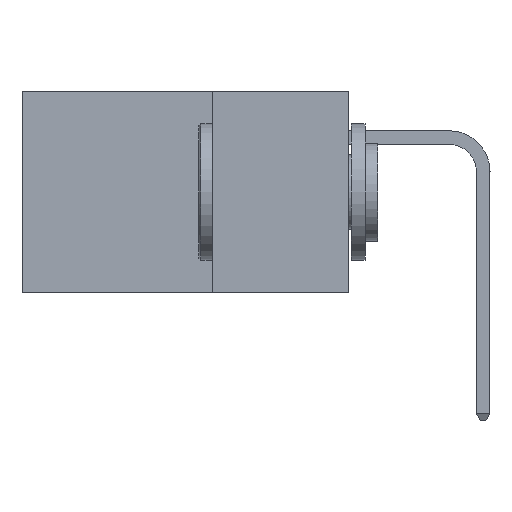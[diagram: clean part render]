
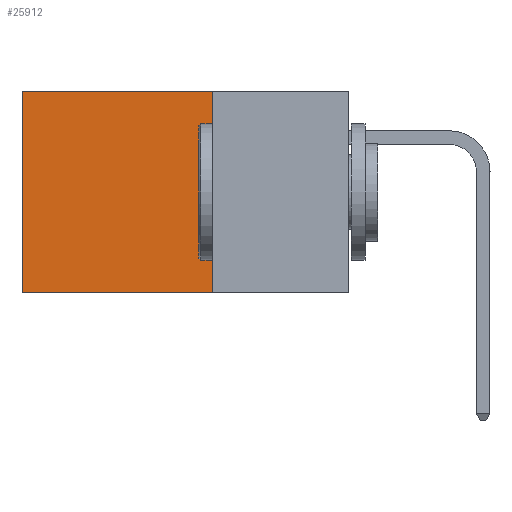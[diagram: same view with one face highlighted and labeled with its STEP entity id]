
A CAD part, left-side view. The second image highlights one B-rep face of the part: STEP entity #25912.
In plain terms, the highlighted planar face has unit normal (-1, 0, 0).
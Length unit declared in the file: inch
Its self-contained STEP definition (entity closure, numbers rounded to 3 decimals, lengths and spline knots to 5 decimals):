
#40 = FACE_OUTER_BOUND ( 'NONE', #26652, .T. ) ;
#1575 = CARTESIAN_POINT ( 'NONE',  ( 0.2875, 0.25, -0.37 ) ) ;
#2164 = VECTOR ( 'NONE', #14780, 39.37008 ) ;
#4225 = CARTESIAN_POINT ( 'NONE',  ( 0.2875, 0.6, 0. ) ) ;
#4243 = DIRECTION ( 'NONE',  ( 1., 0., 0. ) ) ;
#5872 = VERTEX_POINT ( 'NONE', #36141 ) ;
#5880 = VERTEX_POINT ( 'NONE', #33417 ) ;
#5999 = LINE ( 'NONE', #28860, #35302 ) ;
#6138 = VERTEX_POINT ( 'NONE', #14940 ) ;
#9954 = DIRECTION ( 'NONE',  ( 0., 0., -1. ) ) ;
#11559 = VECTOR ( 'NONE', #9954, 39.37008 ) ;
#11646 = ORIENTED_EDGE ( 'NONE', *, *, #27836, .F. ) ;
#11903 = CARTESIAN_POINT ( 'NONE',  ( 0.2875, 0.25, 0. ) ) ;
#14102 = LINE ( 'NONE', #1575, #28128 ) ;
#14710 = AXIS2_PLACEMENT_3D ( 'NONE', #21534, #4243, #24327 ) ;
#14780 = DIRECTION ( 'NONE',  ( 0., 0., -1. ) ) ;
#14940 = CARTESIAN_POINT ( 'NONE',  ( 0.2875, 0.25, 0. ) ) ;
#15315 = ORIENTED_EDGE ( 'NONE', *, *, #17483, .T. ) ;
#17483 = EDGE_CURVE ( 'NONE', #5872, #29052, #26513, .T. ) ;
#17976 = ORIENTED_EDGE ( 'NONE', *, *, #34341, .F. ) ;
#21534 = CARTESIAN_POINT ( 'NONE',  ( 0.2875, 0.25, 0. ) ) ;
#24327 = DIRECTION ( 'NONE',  ( 0., 0., -1. ) ) ;
#24574 = DIRECTION ( 'NONE',  ( 0., 1., 0. ) ) ;
#25063 = LINE ( 'NONE', #11903, #2164 ) ;
#25912 = ADVANCED_FACE ( 'NONE', ( #40 ), #29843, .F. ) ;
#26513 = LINE ( 'NONE', #4225, #11559 ) ;
#26652 = EDGE_LOOP ( 'NONE', ( #15315, #11646, #17976, #30438 ) ) ;
#27836 = EDGE_CURVE ( 'NONE', #5880, #29052, #14102, .T. ) ;
#28128 = VECTOR ( 'NONE', #24574, 39.37008 ) ;
#28860 = CARTESIAN_POINT ( 'NONE',  ( 0.2875, 0.25, 0. ) ) ;
#29052 = VERTEX_POINT ( 'NONE', #34158 ) ;
#29843 = PLANE ( 'NONE',  #14710 ) ;
#30438 = ORIENTED_EDGE ( 'NONE', *, *, #32330, .T. ) ;
#31669 = DIRECTION ( 'NONE',  ( 0., 1., 0. ) ) ;
#32330 = EDGE_CURVE ( 'NONE', #6138, #5872, #5999, .T. ) ;
#33417 = CARTESIAN_POINT ( 'NONE',  ( 0.2875, 0.25, -0.37 ) ) ;
#34158 = CARTESIAN_POINT ( 'NONE',  ( 0.2875, 0.6, -0.37 ) ) ;
#34341 = EDGE_CURVE ( 'NONE', #6138, #5880, #25063, .T. ) ;
#35302 = VECTOR ( 'NONE', #31669, 39.37008 ) ;
#36141 = CARTESIAN_POINT ( 'NONE',  ( 0.2875, 0.6, 0. ) ) ;
